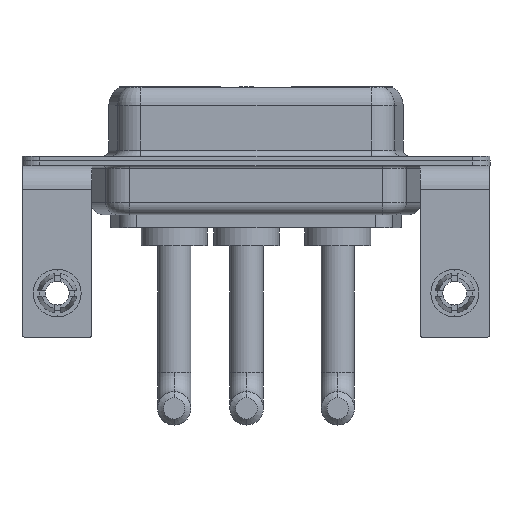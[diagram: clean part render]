
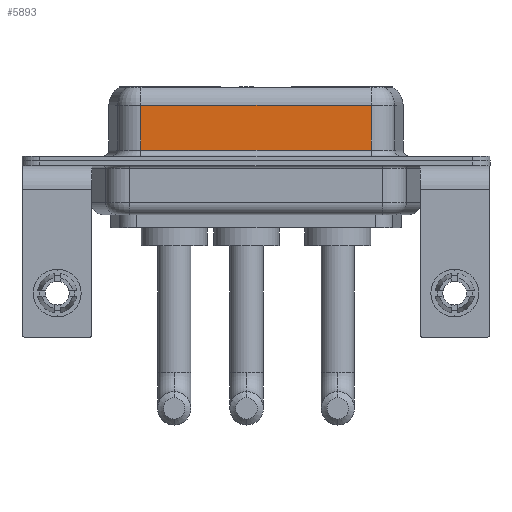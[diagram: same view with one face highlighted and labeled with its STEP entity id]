
A CAD part, front view. The second image highlights one B-rep face of the part: STEP entity #5893.
In plain terms, the highlighted planar face has unit normal (0, -1, 0).
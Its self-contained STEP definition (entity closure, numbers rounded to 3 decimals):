
#237 = FACE_OUTER_BOUND ( 'NONE', #1192, .T. ) ;
#372 = CARTESIAN_POINT ( 'NONE',  ( 26.287, -3.95, 6.4 ) ) ;
#459 = PLANE ( 'NONE',  #2938 ) ;
#625 = VECTOR ( 'NONE', #14618, 1000. ) ;
#861 = VERTEX_POINT ( 'NONE', #5462 ) ;
#1101 = ORIENTED_EDGE ( 'NONE', *, *, #5355, .T. ) ;
#1192 = EDGE_LOOP ( 'NONE', ( #7397, #1484, #16003, #1101 ) ) ;
#1484 = ORIENTED_EDGE ( 'NONE', *, *, #8372, .T. ) ;
#1670 = LINE ( 'NONE', #7641, #10021 ) ;
#2911 = CARTESIAN_POINT ( 'NONE',  ( 26.287, -3.95, 6.4 ) ) ;
#2938 = AXIS2_PLACEMENT_3D ( 'NONE', #2911, #14297, #12824 ) ;
#4046 = DIRECTION ( 'NONE',  ( 0., 0., -1. ) ) ;
#4741 = CARTESIAN_POINT ( 'NONE',  ( 26.287, -3.95, 0.9 ) ) ;
#5096 = CARTESIAN_POINT ( 'NONE',  ( 26.287, -3.95, 0.9 ) ) ;
#5277 = LINE ( 'NONE', #372, #5357 ) ;
#5355 = EDGE_CURVE ( 'NONE', #861, #14198, #11118, .T. ) ;
#5357 = VECTOR ( 'NONE', #4046, 1000. ) ;
#5462 = CARTESIAN_POINT ( 'NONE',  ( 7.013, -3.95, 0.9 ) ) ;
#5893 = ADVANCED_FACE ( 'NONE', ( #237 ), #459, .F. ) ;
#6048 = DIRECTION ( 'NONE',  ( 1., 0., 0. ) ) ;
#6072 = CARTESIAN_POINT ( 'NONE',  ( 26.287, -3.95, 4.65 ) ) ;
#7102 = VECTOR ( 'NONE', #6048, 1000. ) ;
#7397 = ORIENTED_EDGE ( 'NONE', *, *, #15908, .F. ) ;
#7641 = CARTESIAN_POINT ( 'NONE',  ( 26.287, -3.95, 4.65 ) ) ;
#8372 = EDGE_CURVE ( 'NONE', #8824, #11819, #1670, .T. ) ;
#8698 = EDGE_CURVE ( 'NONE', #11819, #861, #15858, .T. ) ;
#8819 = CARTESIAN_POINT ( 'NONE',  ( 7.013, -3.95, 4.65 ) ) ;
#8824 = VERTEX_POINT ( 'NONE', #6072 ) ;
#9589 = CARTESIAN_POINT ( 'NONE',  ( 7.013, -3.95, 6.4 ) ) ;
#10021 = VECTOR ( 'NONE', #10348, 1000. ) ;
#10348 = DIRECTION ( 'NONE',  ( -1., 0., 0. ) ) ;
#11118 = LINE ( 'NONE', #4741, #7102 ) ;
#11819 = VERTEX_POINT ( 'NONE', #8819 ) ;
#12824 = DIRECTION ( 'NONE',  ( 0., 0., 1. ) ) ;
#14198 = VERTEX_POINT ( 'NONE', #5096 ) ;
#14297 = DIRECTION ( 'NONE',  ( 0., 1., 0. ) ) ;
#14618 = DIRECTION ( 'NONE',  ( 0., 0., -1. ) ) ;
#15858 = LINE ( 'NONE', #9589, #625 ) ;
#15908 = EDGE_CURVE ( 'NONE', #8824, #14198, #5277, .T. ) ;
#16003 = ORIENTED_EDGE ( 'NONE', *, *, #8698, .T. ) ;
